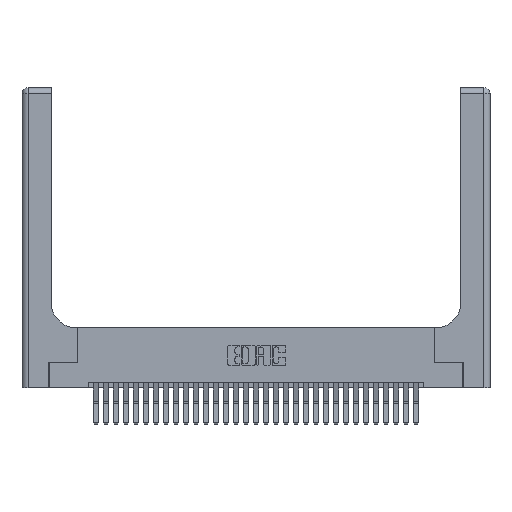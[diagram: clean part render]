
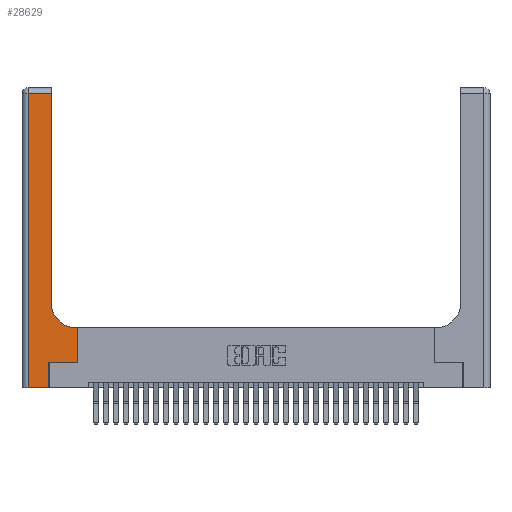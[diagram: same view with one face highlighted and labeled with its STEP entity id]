
A CAD part, top view. The second image highlights one B-rep face of the part: STEP entity #28629.
In plain terms, the highlighted planar face has unit normal (0, 0, 1).
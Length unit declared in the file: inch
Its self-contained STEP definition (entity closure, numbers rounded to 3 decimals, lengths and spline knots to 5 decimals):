
#1356 = LINE ( 'NONE', #26688, #1744 ) ;
#1543 = CARTESIAN_POINT ( 'NONE',  ( 0.2915, 3., 0.37 ) ) ;
#1744 = VECTOR ( 'NONE', #14611, 39.37008 ) ;
#1803 = DIRECTION ( 'NONE',  ( 1., 0., 0. ) ) ;
#3627 = VECTOR ( 'NONE', #12162, 39.37008 ) ;
#3804 = ORIENTED_EDGE ( 'NONE', *, *, #25700, .T. ) ;
#3908 = CARTESIAN_POINT ( 'NONE',  ( 0.5415, 0.85, 0.37 ) ) ;
#5237 = CARTESIAN_POINT ( 'NONE',  ( 0.5585, 0.6, 0.37 ) ) ;
#5459 = LINE ( 'NONE', #27424, #30500 ) ;
#5903 = LINE ( 'NONE', #1543, #17994 ) ;
#6012 = EDGE_CURVE ( 'NONE', #32346, #19698, #10672, .T. ) ;
#6876 = VERTEX_POINT ( 'NONE', #10805 ) ;
#6933 = CARTESIAN_POINT ( 'NONE',  ( 0.269, 0.25, 0.37 ) ) ;
#7006 = CARTESIAN_POINT ( 'NONE',  ( 0.5585, 0.25, 0.37 ) ) ;
#7046 = CARTESIAN_POINT ( 'NONE',  ( 0.2915, 2.94, 0.37 ) ) ;
#7048 = DIRECTION ( 'NONE',  ( 0., 1., 0. ) ) ;
#7201 = VECTOR ( 'NONE', #14188, 39.37008 ) ;
#7623 = CARTESIAN_POINT ( 'NONE',  ( 0.5415, 0.6, 0.37 ) ) ;
#7724 = ORIENTED_EDGE ( 'NONE', *, *, #6012, .T. ) ;
#7979 = EDGE_LOOP ( 'NONE', ( #10787, #18874, #7724, #16639, #19405, #17275, #3804, #14068, #24525 ) ) ;
#8265 = EDGE_CURVE ( 'NONE', #20021, #24919, #5903, .T. ) ;
#8542 = AXIS2_PLACEMENT_3D ( 'NONE', #32207, #31884, #16777 ) ;
#9142 = EDGE_CURVE ( 'NONE', #6876, #23432, #26175, .T. ) ;
#9798 = VERTEX_POINT ( 'NONE', #7623 ) ;
#9960 = EDGE_CURVE ( 'NONE', #19698, #26343, #5459, .T. ) ;
#10108 = CARTESIAN_POINT ( 'NONE',  ( 0.269, 0., 0.37 ) ) ;
#10600 = AXIS2_PLACEMENT_3D ( 'NONE', #3908, #27219, #12171 ) ;
#10672 = LINE ( 'NONE', #11674, #7201 ) ;
#10787 = ORIENTED_EDGE ( 'NONE', *, *, #8265, .T. ) ;
#10805 = CARTESIAN_POINT ( 'NONE',  ( 0.269, 0.25, 0.37 ) ) ;
#11674 = CARTESIAN_POINT ( 'NONE',  ( 0.06, 3., 0.37 ) ) ;
#12162 = DIRECTION ( 'NONE',  ( -1., 0., 0. ) ) ;
#12171 = DIRECTION ( 'NONE',  ( 1., 0., 0. ) ) ;
#12263 = VECTOR ( 'NONE', #7048, 39.37008 ) ;
#13007 = EDGE_CURVE ( 'NONE', #9798, #20021, #28798, .T. ) ;
#13158 = CARTESIAN_POINT ( 'NONE',  ( 0.2915, 0.85, 0.37 ) ) ;
#14068 = ORIENTED_EDGE ( 'NONE', *, *, #15000, .T. ) ;
#14112 = FACE_OUTER_BOUND ( 'NONE', #7979, .T. ) ;
#14188 = DIRECTION ( 'NONE',  ( 0., -1., 0. ) ) ;
#14381 = CARTESIAN_POINT ( 'NONE',  ( 0.06, 0., 0.37 ) ) ;
#14611 = DIRECTION ( 'NONE',  ( -1., 0., 0. ) ) ;
#14893 = DIRECTION ( 'NONE',  ( 1., 0., 0. ) ) ;
#15000 = EDGE_CURVE ( 'NONE', #30141, #9798, #29857, .T. ) ;
#16639 = ORIENTED_EDGE ( 'NONE', *, *, #9960, .T. ) ;
#16777 = DIRECTION ( 'NONE',  ( -1., 0., 0. ) ) ;
#17096 = CARTESIAN_POINT ( 'NONE',  ( 0.269, 0., 0.37 ) ) ;
#17275 = ORIENTED_EDGE ( 'NONE', *, *, #9142, .T. ) ;
#17641 = CARTESIAN_POINT ( 'NONE',  ( 0.2915, 0.6, 0.37 ) ) ;
#17994 = VECTOR ( 'NONE', #31049, 39.37008 ) ;
#18874 = ORIENTED_EDGE ( 'NONE', *, *, #30588, .T. ) ;
#19405 = ORIENTED_EDGE ( 'NONE', *, *, #26675, .T. ) ;
#19572 = DIRECTION ( 'NONE',  ( 0., 1., 0. ) ) ;
#19698 = VERTEX_POINT ( 'NONE', #14381 ) ;
#20021 = VERTEX_POINT ( 'NONE', #13158 ) ;
#20983 = VECTOR ( 'NONE', #19572, 39.37008 ) ;
#22932 = LINE ( 'NONE', #7006, #20983 ) ;
#23043 = CARTESIAN_POINT ( 'NONE',  ( 0.5585, 0.25, 0.37 ) ) ;
#23432 = VERTEX_POINT ( 'NONE', #23043 ) ;
#24182 = CARTESIAN_POINT ( 'NONE',  ( 0.06, 2.94, 0.37 ) ) ;
#24525 = ORIENTED_EDGE ( 'NONE', *, *, #13007, .T. ) ;
#24919 = VERTEX_POINT ( 'NONE', #7046 ) ;
#25700 = EDGE_CURVE ( 'NONE', #23432, #30141, #22932, .T. ) ;
#26032 = LINE ( 'NONE', #17096, #12263 ) ;
#26175 = LINE ( 'NONE', #6933, #28906 ) ;
#26343 = VERTEX_POINT ( 'NONE', #10108 ) ;
#26675 = EDGE_CURVE ( 'NONE', #26343, #6876, #26032, .T. ) ;
#26688 = CARTESIAN_POINT ( 'NONE',  ( 0., 2.94, 0.37 ) ) ;
#27219 = DIRECTION ( 'NONE',  ( 0., 0., -1. ) ) ;
#27424 = CARTESIAN_POINT ( 'NONE',  ( 0., 0., 0.37 ) ) ;
#28629 = ADVANCED_FACE ( 'NONE', ( #14112 ), #31785, .F. ) ;
#28798 = CIRCLE ( 'NONE', #10600, 0.25 ) ;
#28906 = VECTOR ( 'NONE', #1803, 39.37008 ) ;
#29857 = LINE ( 'NONE', #17641, #3627 ) ;
#30141 = VERTEX_POINT ( 'NONE', #5237 ) ;
#30500 = VECTOR ( 'NONE', #14893, 39.37008 ) ;
#30588 = EDGE_CURVE ( 'NONE', #24919, #32346, #1356, .T. ) ;
#31049 = DIRECTION ( 'NONE',  ( 0., 1., 0. ) ) ;
#31785 = PLANE ( 'NONE',  #8542 ) ;
#31884 = DIRECTION ( 'NONE',  ( 0., 0., -1. ) ) ;
#32207 = CARTESIAN_POINT ( 'NONE',  ( 0., 3., 0.37 ) ) ;
#32346 = VERTEX_POINT ( 'NONE', #24182 ) ;
